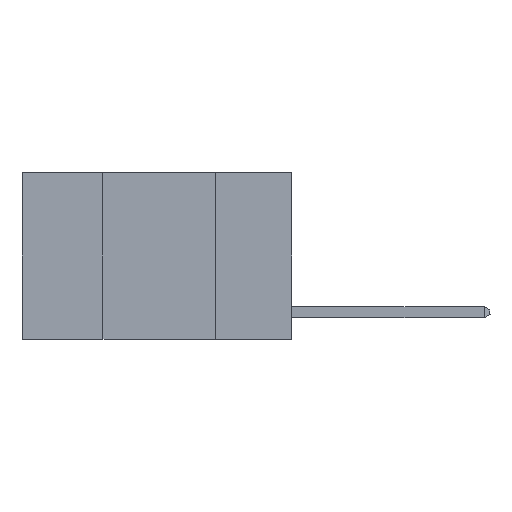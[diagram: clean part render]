
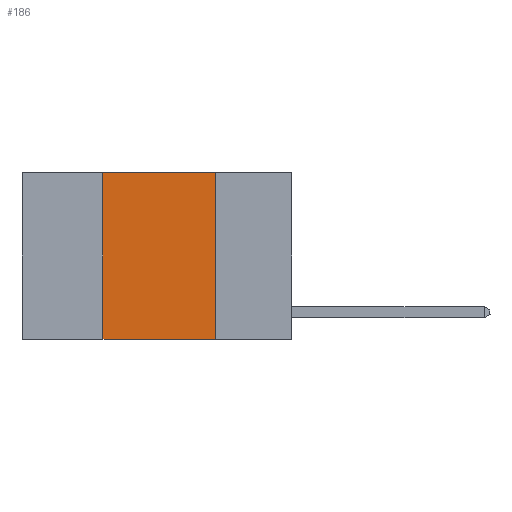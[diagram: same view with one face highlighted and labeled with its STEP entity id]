
A CAD part, left-side view. The second image highlights one B-rep face of the part: STEP entity #186.
In plain terms, the highlighted planar face has unit normal (-1, 0, 0).
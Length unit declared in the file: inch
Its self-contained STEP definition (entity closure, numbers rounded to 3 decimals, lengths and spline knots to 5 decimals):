
#133 = CARTESIAN_POINT ( 'NONE',  ( 0., 0.6, 0. ) ) ;
#186 = ADVANCED_FACE ( 'NONE', ( #12802 ), #7141, .F. ) ;
#2976 = EDGE_CURVE ( 'NONE', #5040, #8156, #8237, .T. ) ;
#3186 = DIRECTION ( 'NONE',  ( 0., 0., 1. ) ) ;
#3695 = CARTESIAN_POINT ( 'NONE',  ( 0., 0.42, -0.37 ) ) ;
#3721 = DIRECTION ( 'NONE',  ( 0., 0., -1. ) ) ;
#3724 = LINE ( 'NONE', #133, #22724 ) ;
#4114 = VERTEX_POINT ( 'NONE', #8931 ) ;
#4117 = ORIENTED_EDGE ( 'NONE', *, *, #6021, .F. ) ;
#5040 = VERTEX_POINT ( 'NONE', #3695 ) ;
#5294 = DIRECTION ( 'NONE',  ( 0., -1., 0. ) ) ;
#6021 = EDGE_CURVE ( 'NONE', #5040, #4114, #17593, .T. ) ;
#6784 = CARTESIAN_POINT ( 'NONE',  ( 0., 0.42, 0. ) ) ;
#7141 = PLANE ( 'NONE',  #17392 ) ;
#7605 = VECTOR ( 'NONE', #3721, 39.37008 ) ;
#7824 = EDGE_LOOP ( 'NONE', ( #8131, #20275, #4117, #19066 ) ) ;
#8131 = ORIENTED_EDGE ( 'NONE', *, *, #16138, .F. ) ;
#8156 = VERTEX_POINT ( 'NONE', #11028 ) ;
#8237 = LINE ( 'NONE', #14001, #21114 ) ;
#8922 = DIRECTION ( 'NONE',  ( 0., 0., -1. ) ) ;
#8931 = CARTESIAN_POINT ( 'NONE',  ( 0., 0.42, 0. ) ) ;
#9868 = CARTESIAN_POINT ( 'NONE',  ( 0., 0.17, 0. ) ) ;
#10635 = DIRECTION ( 'NONE',  ( 1., 0., 0. ) ) ;
#11028 = CARTESIAN_POINT ( 'NONE',  ( 0., 0.17, -0.37 ) ) ;
#11753 = DIRECTION ( 'NONE',  ( 0., -1., 0. ) ) ;
#12512 = LINE ( 'NONE', #20239, #7605 ) ;
#12802 = FACE_OUTER_BOUND ( 'NONE', #7824, .T. ) ;
#14001 = CARTESIAN_POINT ( 'NONE',  ( 0., 0.6, -0.37 ) ) ;
#14854 = VECTOR ( 'NONE', #3186, 39.37008 ) ;
#16138 = EDGE_CURVE ( 'NONE', #20219, #8156, #12512, .T. ) ;
#17392 = AXIS2_PLACEMENT_3D ( 'NONE', #23400, #10635, #8922 ) ;
#17593 = LINE ( 'NONE', #6784, #14854 ) ;
#19066 = ORIENTED_EDGE ( 'NONE', *, *, #2976, .T. ) ;
#20219 = VERTEX_POINT ( 'NONE', #9868 ) ;
#20239 = CARTESIAN_POINT ( 'NONE',  ( 0., 0.17, 0. ) ) ;
#20275 = ORIENTED_EDGE ( 'NONE', *, *, #21343, .F. ) ;
#21114 = VECTOR ( 'NONE', #11753, 39.37008 ) ;
#21343 = EDGE_CURVE ( 'NONE', #4114, #20219, #3724, .T. ) ;
#22724 = VECTOR ( 'NONE', #5294, 39.37008 ) ;
#23400 = CARTESIAN_POINT ( 'NONE',  ( 0., 0.6, 0. ) ) ;
